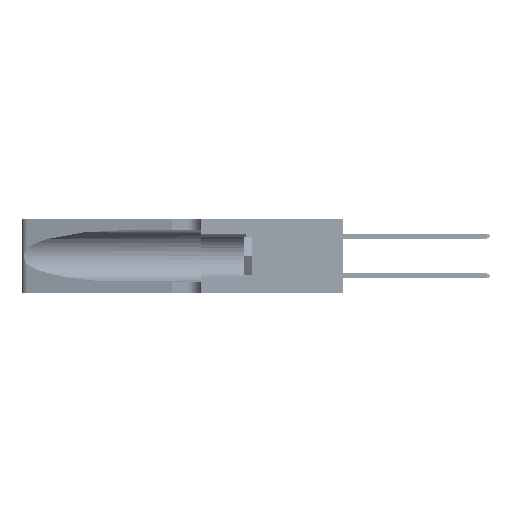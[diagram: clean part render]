
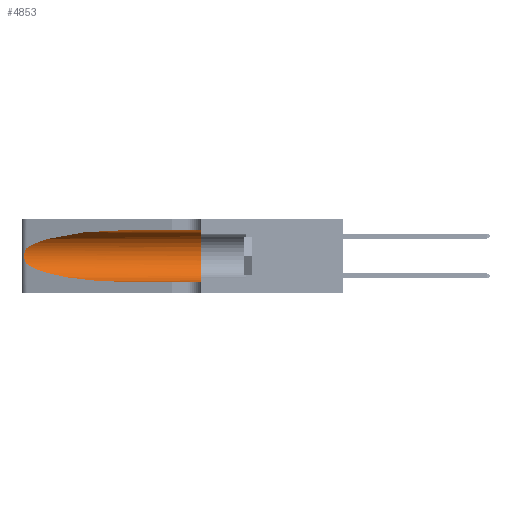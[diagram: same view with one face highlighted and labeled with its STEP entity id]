
A CAD part, left-side view. The second image highlights one B-rep face of the part: STEP entity #4853.
In plain terms, the highlighted cylindrical face has radius 3.308 mm (diameter 6.617 mm), a partial arc.
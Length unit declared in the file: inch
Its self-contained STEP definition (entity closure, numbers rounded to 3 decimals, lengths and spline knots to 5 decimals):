
#16 = CARTESIAN_POINT ( 'NONE',  ( 0.25487, 1.22718, 0.22369 ) ) ;
#692 = CARTESIAN_POINT ( 'NONE',  ( 0.25856, 1.23593, 0.16098 ) ) ;
#885 = CARTESIAN_POINT ( 'NONE',  ( 0.26075, 1.23896, 0.178 ) ) ;
#3071 = DIRECTION ( 'NONE',  ( 0., 0., -1. ) ) ;
#3531 = VERTEX_POINT ( 'NONE', #54064 ) ;
#4853 = ADVANCED_FACE ( 'NONE', ( #51172 ), #20070, .F. ) ;
#5095 = CARTESIAN_POINT ( 'NONE',  ( 0.25639, 1.23186, 0.15144 ) ) ;
#5875 = AXIS2_PLACEMENT_3D ( 'NONE', #38154, #12519, #38344 ) ;
#6222 = EDGE_CURVE ( 'NONE', #49991, #32176, #45097, .T. ) ;
#6454 = DIRECTION ( 'NONE',  ( 0., -1., 0. ) ) ;
#6693 = VECTOR ( 'NONE', #6454, 39.37008 ) ;
#6781 = LINE ( 'NONE', #27945, #39290 ) ;
#7514 = CARTESIAN_POINT ( 'NONE',  ( 0.1305, 0.72297, 0.31525 ) ) ;
#7942 = CARTESIAN_POINT ( 'NONE',  ( 0.18966, 0.96281, 0.31525 ) ) ;
#11702 = EDGE_CURVE ( 'NONE', #17786, #27291, #26622, .T. ) ;
#12519 = DIRECTION ( 'NONE',  ( 0., 1., 0. ) ) ;
#13404 = CARTESIAN_POINT ( 'NONE',  ( 0.25487, 1.22718, 0.14631 ) ) ;
#13821 = EDGE_CURVE ( 'NONE', #27291, #3531, #20811, .T. ) ;
#14392 = ORIENTED_EDGE ( 'NONE', *, *, #15415, .F. ) ;
#14957 = ORIENTED_EDGE ( 'NONE', *, *, #49077, .T. ) ;
#15415 = EDGE_CURVE ( 'NONE', #51499, #49991, #6781, .T. ) ;
#17680 = CARTESIAN_POINT ( 'NONE',  ( 0.25639, 1.23184, 0.21858 ) ) ;
#17786 = VERTEX_POINT ( 'NONE', #26809 ) ;
#20070 = CYLINDRICAL_SURFACE ( 'NONE', #44165, 0.13025 ) ;
#20575 = CARTESIAN_POINT ( 'NONE',  ( 0.1305, 0.72297, 0.31525 ) ) ;
#20811 =( BOUNDED_CURVE ( )  B_SPLINE_CURVE ( 3, ( #21475, #25199, #38156, #42412 ),
 .UNSPECIFIED., .F., .F. ) 
 B_SPLINE_CURVE_WITH_KNOTS ( ( 4, 4 ),
 ( 3.44316, 4.71239 ),
 .UNSPECIFIED. ) 
 CURVE ( )  GEOMETRIC_REPRESENTATION_ITEM ( )  RATIONAL_B_SPLINE_CURVE ( ( 1., 0.87, 0.87, 1. ) ) 
 REPRESENTATION_ITEM ( '' )  );
#21426 = ORIENTED_EDGE ( 'NONE', *, *, #11702, .T. ) ;
#21475 = CARTESIAN_POINT ( 'NONE',  ( 0.25487, 1.22718, 0.14631 ) ) ;
#21743 = CARTESIAN_POINT ( 'NONE',  ( 0.1305, 0.35, 0.31525 ) ) ;
#22164 = CARTESIAN_POINT ( 'NONE',  ( 0.26075, 1.23896, 0.19203 ) ) ;
#22518 =( BOUNDED_CURVE ( )  B_SPLINE_CURVE ( 3, ( #20575, #7942, #33936, #16 ),
 .UNSPECIFIED., .F., .F. ) 
 B_SPLINE_CURVE_WITH_KNOTS ( ( 4, 4 ),
 ( 1.5708, 2.84003 ),
 .UNSPECIFIED. ) 
 CURVE ( )  GEOMETRIC_REPRESENTATION_ITEM ( )  RATIONAL_B_SPLINE_CURVE ( ( 1., 0.87, 0.87, 1. ) ) 
 REPRESENTATION_ITEM ( '' )  );
#24201 = CARTESIAN_POINT ( 'NONE',  ( 0.1305, 1.61858, 0.185 ) ) ;
#25199 = CARTESIAN_POINT ( 'NONE',  ( 0.2373, 1.15595, 0.08982 ) ) ;
#26077 = CARTESIAN_POINT ( 'NONE',  ( 0.25555, 1.22994, 0.2215 ) ) ;
#26622 = B_SPLINE_CURVE_WITH_KNOTS ( 'NONE', 3,
 ( #47852, #26077, #17680, #34780, #43094, #30718, #22164, #885, #47666, #692, #34606, #5095, #51742, #13404 ),
 .UNSPECIFIED., .F., .F.,
 ( 4, 2, 2, 2, 2, 2, 4 ),
 ( 0., 0.00027, 0.00053, 0.00107, 0.0016, 0.00187, 0.00214 ),
 .UNSPECIFIED. ) ;
#26809 = CARTESIAN_POINT ( 'NONE',  ( 0.25487, 1.22718, 0.22369 ) ) ;
#27066 = EDGE_LOOP ( 'NONE', ( #51393, #21426, #29004, #14957, #41776, #14392 ) ) ;
#27291 = VERTEX_POINT ( 'NONE', #51073 ) ;
#27945 = CARTESIAN_POINT ( 'NONE',  ( 0.1305, 1.61858, 0.31525 ) ) ;
#29004 = ORIENTED_EDGE ( 'NONE', *, *, #13821, .T. ) ;
#30718 = CARTESIAN_POINT ( 'NONE',  ( 0.26018, 1.23835, 0.19895 ) ) ;
#31180 = EDGE_CURVE ( 'NONE', #51499, #17786, #22518, .T. ) ;
#32176 = VERTEX_POINT ( 'NONE', #52075 ) ;
#33936 = CARTESIAN_POINT ( 'NONE',  ( 0.2373, 1.15595, 0.28018 ) ) ;
#34606 = CARTESIAN_POINT ( 'NONE',  ( 0.25789, 1.23486, 0.15765 ) ) ;
#34780 = CARTESIAN_POINT ( 'NONE',  ( 0.25787, 1.23484, 0.2124 ) ) ;
#38154 = CARTESIAN_POINT ( 'NONE',  ( 0.1305, 0.35, 0.185 ) ) ;
#38156 = CARTESIAN_POINT ( 'NONE',  ( 0.18966, 0.96281, 0.05475 ) ) ;
#38344 = DIRECTION ( 'NONE',  ( 0., 0., 1. ) ) ;
#39290 = VECTOR ( 'NONE', #49721, 39.37008 ) ;
#40738 = CARTESIAN_POINT ( 'NONE',  ( 0.1305, 1.61858, 0.05475 ) ) ;
#41776 = ORIENTED_EDGE ( 'NONE', *, *, #6222, .F. ) ;
#41840 = LINE ( 'NONE', #40738, #6693 ) ;
#42412 = CARTESIAN_POINT ( 'NONE',  ( 0.1305, 0.72297, 0.05475 ) ) ;
#43094 = CARTESIAN_POINT ( 'NONE',  ( 0.25854, 1.2359, 0.20912 ) ) ;
#44165 = AXIS2_PLACEMENT_3D ( 'NONE', #24201, #53748, #3071 ) ;
#45097 = CIRCLE ( 'NONE', #5875, 0.13025 ) ;
#47666 = CARTESIAN_POINT ( 'NONE',  ( 0.26017, 1.23833, 0.17102 ) ) ;
#47852 = CARTESIAN_POINT ( 'NONE',  ( 0.25487, 1.22718, 0.22369 ) ) ;
#49077 = EDGE_CURVE ( 'NONE', #3531, #32176, #41840, .T. ) ;
#49721 = DIRECTION ( 'NONE',  ( 0., -1., 0. ) ) ;
#49991 = VERTEX_POINT ( 'NONE', #21743 ) ;
#51073 = CARTESIAN_POINT ( 'NONE',  ( 0.25487, 1.22718, 0.14631 ) ) ;
#51172 = FACE_OUTER_BOUND ( 'NONE', #27066, .T. ) ;
#51393 = ORIENTED_EDGE ( 'NONE', *, *, #31180, .T. ) ;
#51499 = VERTEX_POINT ( 'NONE', #7514 ) ;
#51742 = CARTESIAN_POINT ( 'NONE',  ( 0.25555, 1.22993, 0.14849 ) ) ;
#52075 = CARTESIAN_POINT ( 'NONE',  ( 0.1305, 0.35, 0.05475 ) ) ;
#53748 = DIRECTION ( 'NONE',  ( 0., -1., 0. ) ) ;
#54064 = CARTESIAN_POINT ( 'NONE',  ( 0.1305, 0.72297, 0.05475 ) ) ;
